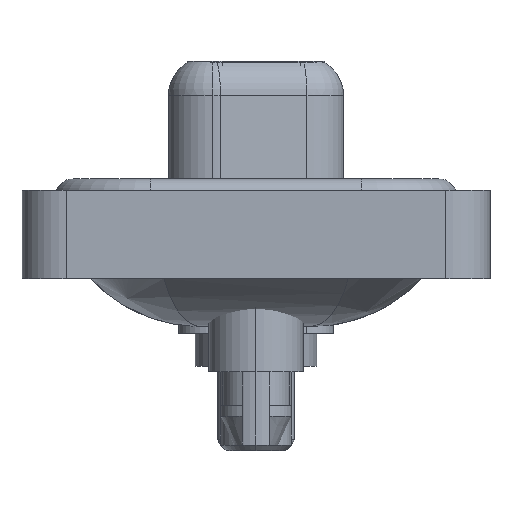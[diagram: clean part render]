
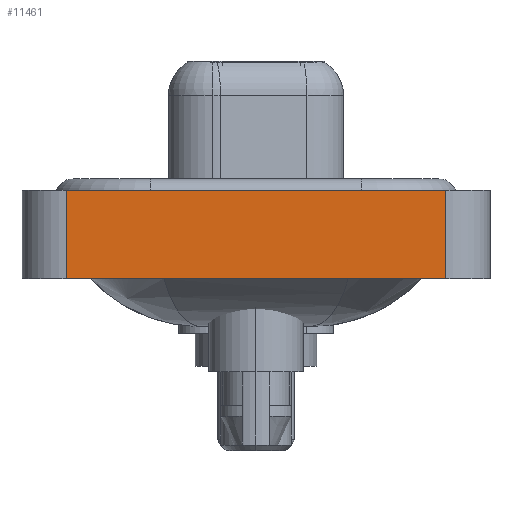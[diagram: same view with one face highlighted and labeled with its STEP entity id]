
A CAD part, left-side view. The second image highlights one B-rep face of the part: STEP entity #11461.
In plain terms, the highlighted planar face has unit normal (-1, 0, 0).
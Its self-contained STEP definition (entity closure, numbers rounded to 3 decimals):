
#669 = DIRECTION ( 'NONE',  ( 0., -1., 0. ) ) ;
#1482 = ORIENTED_EDGE ( 'NONE', *, *, #6495, .F. ) ;
#1834 = DIRECTION ( 'NONE',  ( -1., 0., 0. ) ) ;
#2090 = CARTESIAN_POINT ( 'NONE',  ( -7.3, 8.55, 0.4 ) ) ;
#2098 = AXIS2_PLACEMENT_3D ( 'NONE', #16741, #1834, #10046 ) ;
#3559 = PLANE ( 'NONE',  #2098 ) ;
#4708 = DIRECTION ( 'NONE',  ( 0., 0., 1. ) ) ;
#4792 = VERTEX_POINT ( 'NONE', #2090 ) ;
#5098 = ORIENTED_EDGE ( 'NONE', *, *, #21192, .F. ) ;
#5261 = FACE_OUTER_BOUND ( 'NONE', #18013, .T. ) ;
#5760 = VERTEX_POINT ( 'NONE', #14213 ) ;
#5808 = LINE ( 'NONE', #12338, #16891 ) ;
#6495 = EDGE_CURVE ( 'NONE', #4792, #5760, #5808, .T. ) ;
#6603 = DIRECTION ( 'NONE',  ( 0., -1., 0. ) ) ;
#10046 = DIRECTION ( 'NONE',  ( 0., 0., 1. ) ) ;
#10245 = VERTEX_POINT ( 'NONE', #18955 ) ;
#11178 = CARTESIAN_POINT ( 'NONE',  ( -7.3, -8.55, -3.6 ) ) ;
#11461 = ADVANCED_FACE ( 'NONE', ( #5261 ), #3559, .T. ) ;
#11913 = LINE ( 'NONE', #15163, #15855 ) ;
#12338 = CARTESIAN_POINT ( 'NONE',  ( -7.3, -8.55, 0.4 ) ) ;
#14213 = CARTESIAN_POINT ( 'NONE',  ( -7.3, -8.55, 0.4 ) ) ;
#15163 = CARTESIAN_POINT ( 'NONE',  ( -7.3, 8.55, -3.6 ) ) ;
#15855 = VECTOR ( 'NONE', #19669, 1000. ) ;
#16315 = CARTESIAN_POINT ( 'NONE',  ( -7.3, 8.55, -3.6 ) ) ;
#16413 = LINE ( 'NONE', #19717, #19900 ) ;
#16741 = CARTESIAN_POINT ( 'NONE',  ( -7.3, -8.55, -3.6 ) ) ;
#16891 = VECTOR ( 'NONE', #669, 1000. ) ;
#17434 = ORIENTED_EDGE ( 'NONE', *, *, #20403, .T. ) ;
#17873 = VERTEX_POINT ( 'NONE', #16315 ) ;
#18013 = EDGE_LOOP ( 'NONE', ( #17434, #1482, #5098, #20286 ) ) ;
#18955 = CARTESIAN_POINT ( 'NONE',  ( -7.3, -8.55, -3.6 ) ) ;
#19477 = LINE ( 'NONE', #11178, #20956 ) ;
#19669 = DIRECTION ( 'NONE',  ( 0., 0., 1. ) ) ;
#19717 = CARTESIAN_POINT ( 'NONE',  ( -7.3, -8.55, -3.6 ) ) ;
#19900 = VECTOR ( 'NONE', #4708, 1000. ) ;
#20286 = ORIENTED_EDGE ( 'NONE', *, *, #20808, .T. ) ;
#20403 = EDGE_CURVE ( 'NONE', #10245, #5760, #16413, .T. ) ;
#20808 = EDGE_CURVE ( 'NONE', #17873, #10245, #19477, .T. ) ;
#20956 = VECTOR ( 'NONE', #6603, 1000. ) ;
#21192 = EDGE_CURVE ( 'NONE', #17873, #4792, #11913, .T. ) ;
